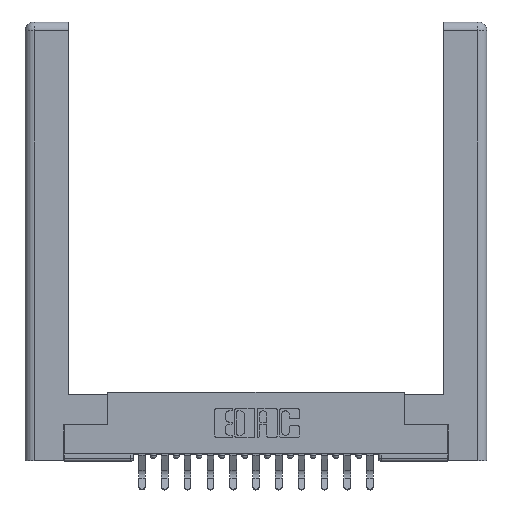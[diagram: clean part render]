
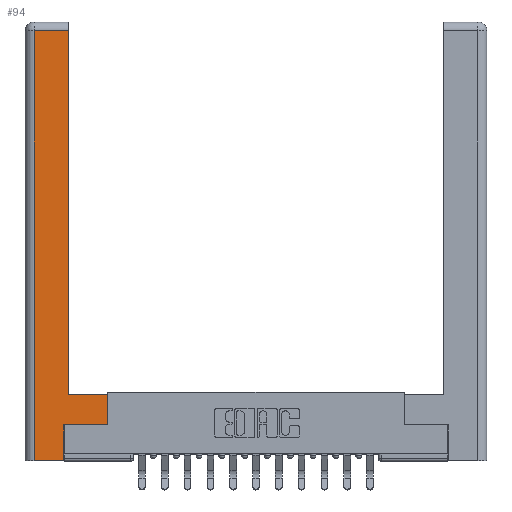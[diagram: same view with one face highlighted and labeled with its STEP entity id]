
A CAD part, top view. The second image highlights one B-rep face of the part: STEP entity #94.
In plain terms, the highlighted planar face has unit normal (0, 0, 1).
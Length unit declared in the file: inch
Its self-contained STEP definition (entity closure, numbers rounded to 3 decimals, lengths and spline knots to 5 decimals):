
#55 = CARTESIAN_POINT ( 'NONE',  ( 0.0615, 0., 0. ) ) ;
#94 = ADVANCED_FACE ( 'NONE', ( #12869 ), #11327, .F. ) ;
#124 = LINE ( 'NONE', #55, #7014 ) ;
#233 = CARTESIAN_POINT ( 'NONE',  ( 0.295, 2.94, 0. ) ) ;
#523 = CARTESIAN_POINT ( 'NONE',  ( 0.265, 0., 0. ) ) ;
#641 = LINE ( 'NONE', #2819, #1605 ) ;
#976 = LINE ( 'NONE', #2830, #12041 ) ;
#1059 = CARTESIAN_POINT ( 'NONE',  ( 0.265, 0.245, 0. ) ) ;
#1295 = VECTOR ( 'NONE', #8165, 39.37008 ) ;
#1557 = VERTEX_POINT ( 'NONE', #1059 ) ;
#1605 = VECTOR ( 'NONE', #5363, 39.37008 ) ;
#1653 = ORIENTED_EDGE ( 'NONE', *, *, #12486, .T. ) ;
#1704 = VECTOR ( 'NONE', #2174, 39.37008 ) ;
#2174 = DIRECTION ( 'NONE',  ( 0., 1., 0. ) ) ;
#2352 = CARTESIAN_POINT ( 'NONE',  ( 0.565, 0.45, 0. ) ) ;
#2606 = LINE ( 'NONE', #6739, #8894 ) ;
#2819 = CARTESIAN_POINT ( 'NONE',  ( 0.295, 3., 0. ) ) ;
#2830 = CARTESIAN_POINT ( 'NONE',  ( 0.0615, 2.94, 0. ) ) ;
#3088 = EDGE_CURVE ( 'NONE', #8873, #14935, #8397, .T. ) ;
#3192 = CARTESIAN_POINT ( 'NONE',  ( 0.295, 0.45, 0. ) ) ;
#3376 = CARTESIAN_POINT ( 'NONE',  ( 0.0615, 2.94, 0. ) ) ;
#3809 = EDGE_CURVE ( 'NONE', #14935, #11737, #7964, .T. ) ;
#4933 = EDGE_CURVE ( 'NONE', #16105, #15420, #976, .T. ) ;
#5023 = ORIENTED_EDGE ( 'NONE', *, *, #14972, .T. ) ;
#5122 = DIRECTION ( 'NONE',  ( -1., 0., 0. ) ) ;
#5363 = DIRECTION ( 'NONE',  ( 0., 1., 0. ) ) ;
#5478 = VERTEX_POINT ( 'NONE', #6699 ) ;
#6599 = EDGE_CURVE ( 'NONE', #15420, #5478, #124, .T. ) ;
#6699 = CARTESIAN_POINT ( 'NONE',  ( 0.0615, 0., 0. ) ) ;
#6739 = CARTESIAN_POINT ( 'NONE',  ( 0.265, 0.245, 0. ) ) ;
#6944 = CARTESIAN_POINT ( 'NONE',  ( 0.565, 0.245, 0. ) ) ;
#7014 = VECTOR ( 'NONE', #14081, 39.37008 ) ;
#7286 = ORIENTED_EDGE ( 'NONE', *, *, #14679, .T. ) ;
#7510 = CARTESIAN_POINT ( 'NONE',  ( 0., 0., 0. ) ) ;
#7658 = CARTESIAN_POINT ( 'NONE',  ( 0.565, 0.245, 0. ) ) ;
#7951 = ORIENTED_EDGE ( 'NONE', *, *, #11927, .T. ) ;
#7964 = LINE ( 'NONE', #3192, #1295 ) ;
#8165 = DIRECTION ( 'NONE',  ( -1., 0., 0. ) ) ;
#8177 = VECTOR ( 'NONE', #12845, 39.37008 ) ;
#8397 = LINE ( 'NONE', #2352, #1704 ) ;
#8777 = DIRECTION ( 'NONE',  ( 0., 0., -1. ) ) ;
#8873 = VERTEX_POINT ( 'NONE', #7658 ) ;
#8893 = CARTESIAN_POINT ( 'NONE',  ( 0.265, 0., 0. ) ) ;
#8894 = VECTOR ( 'NONE', #15761, 39.37008 ) ;
#9003 = ORIENTED_EDGE ( 'NONE', *, *, #3088, .T. ) ;
#9792 = LINE ( 'NONE', #6944, #12419 ) ;
#9876 = CARTESIAN_POINT ( 'NONE',  ( 0.565, 0.45, 0. ) ) ;
#9895 = EDGE_LOOP ( 'NONE', ( #7951, #13810, #10262, #5023, #1653, #7286, #9003, #14329 ) ) ;
#10262 = ORIENTED_EDGE ( 'NONE', *, *, #6599, .T. ) ;
#11327 = PLANE ( 'NONE',  #14008 ) ;
#11534 = DIRECTION ( 'NONE',  ( -1., 0., 0. ) ) ;
#11737 = VERTEX_POINT ( 'NONE', #12720 ) ;
#11927 = EDGE_CURVE ( 'NONE', #11737, #16105, #641, .T. ) ;
#11981 = LINE ( 'NONE', #8893, #8177 ) ;
#12041 = VECTOR ( 'NONE', #11534, 39.37008 ) ;
#12419 = VECTOR ( 'NONE', #13222, 39.37008 ) ;
#12486 = EDGE_CURVE ( 'NONE', #14727, #1557, #2606, .T. ) ;
#12720 = CARTESIAN_POINT ( 'NONE',  ( 0.295, 0.45, 0. ) ) ;
#12845 = DIRECTION ( 'NONE',  ( 1., 0., 0. ) ) ;
#12869 = FACE_OUTER_BOUND ( 'NONE', #9895, .T. ) ;
#13222 = DIRECTION ( 'NONE',  ( 1., 0., 0. ) ) ;
#13810 = ORIENTED_EDGE ( 'NONE', *, *, #4933, .T. ) ;
#14008 = AXIS2_PLACEMENT_3D ( 'NONE', #7510, #8777, #5122 ) ;
#14081 = DIRECTION ( 'NONE',  ( 0., -1., 0. ) ) ;
#14329 = ORIENTED_EDGE ( 'NONE', *, *, #3809, .T. ) ;
#14679 = EDGE_CURVE ( 'NONE', #1557, #8873, #9792, .T. ) ;
#14727 = VERTEX_POINT ( 'NONE', #523 ) ;
#14935 = VERTEX_POINT ( 'NONE', #9876 ) ;
#14972 = EDGE_CURVE ( 'NONE', #5478, #14727, #11981, .T. ) ;
#15420 = VERTEX_POINT ( 'NONE', #3376 ) ;
#15761 = DIRECTION ( 'NONE',  ( 0., 1., 0. ) ) ;
#16105 = VERTEX_POINT ( 'NONE', #233 ) ;
